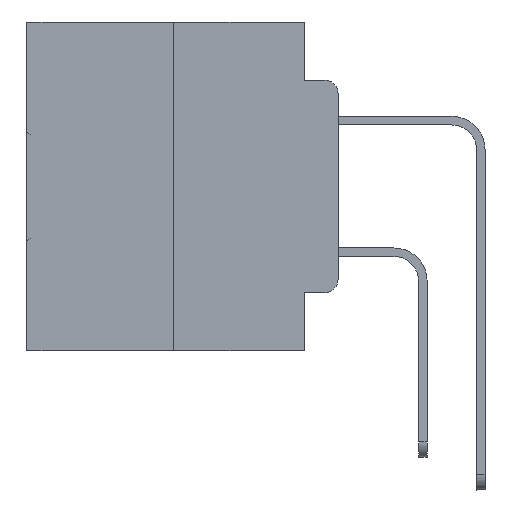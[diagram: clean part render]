
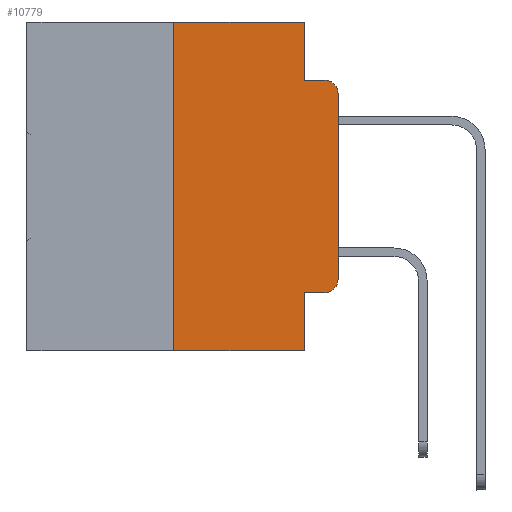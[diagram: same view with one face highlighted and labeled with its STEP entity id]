
A CAD part, left-side view. The second image highlights one B-rep face of the part: STEP entity #10779.
In plain terms, the highlighted planar face has unit normal (-1, 0, 0).
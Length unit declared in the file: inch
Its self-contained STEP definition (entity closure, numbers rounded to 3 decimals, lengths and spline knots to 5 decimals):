
#100 = VERTEX_POINT ( 'NONE', #12382 ) ;
#113 = DIRECTION ( 'NONE',  ( 0., 0., 1. ) ) ;
#302 = LINE ( 'NONE', #7705, #11206 ) ;
#1201 = PLANE ( 'NONE',  #13483 ) ;
#1510 = LINE ( 'NONE', #9770, #7152 ) ;
#1679 = DIRECTION ( 'NONE',  ( 0., -1., 0. ) ) ;
#1878 = CARTESIAN_POINT ( 'NONE',  ( 0., 0.051, 0. ) ) ;
#1931 = VERTEX_POINT ( 'NONE', #5113 ) ;
#3288 = VECTOR ( 'NONE', #32400, 39.37008 ) ;
#3996 = ORIENTED_EDGE ( 'NONE', *, *, #16069, .T. ) ;
#4179 = CARTESIAN_POINT ( 'NONE',  ( 0., 0., -0.1085 ) ) ;
#4691 = VECTOR ( 'NONE', #113, 39.37008 ) ;
#5071 = DIRECTION ( 'NONE',  ( 0., -1., 0. ) ) ;
#5113 = CARTESIAN_POINT ( 'NONE',  ( 0., 0.02, -0.0885 ) ) ;
#5493 = VECTOR ( 'NONE', #5071, 39.37008 ) ;
#6468 = DIRECTION ( 'NONE',  ( 1., 0., 0. ) ) ;
#7084 = CARTESIAN_POINT ( 'NONE',  ( 0., 0.051, -0.4115 ) ) ;
#7152 = VECTOR ( 'NONE', #1679, 39.37008 ) ;
#7705 = CARTESIAN_POINT ( 'NONE',  ( 0., 0., 0. ) ) ;
#8495 = VERTEX_POINT ( 'NONE', #10534 ) ;
#8621 = EDGE_CURVE ( 'NONE', #27660, #28685, #11044, .T. ) ;
#8738 = VERTEX_POINT ( 'NONE', #13031 ) ;
#9267 = DIRECTION ( 'NONE',  ( 0., 0., -1. ) ) ;
#9281 = EDGE_CURVE ( 'NONE', #28875, #8738, #16514, .T. ) ;
#9294 = DIRECTION ( 'NONE',  ( 0., -1., 0. ) ) ;
#9384 = CIRCLE ( 'NONE', #15091, 0.02 ) ;
#9770 = CARTESIAN_POINT ( 'NONE',  ( 0., 0.473, 0. ) ) ;
#9785 = ORIENTED_EDGE ( 'NONE', *, *, #31784, .T. ) ;
#10319 = AXIS2_PLACEMENT_3D ( 'NONE', #24698, #22269, #21919 ) ;
#10534 = CARTESIAN_POINT ( 'NONE',  ( 0., 0.25, -0.5 ) ) ;
#10779 = ADVANCED_FACE ( 'NONE', ( #14029 ), #1201, .F. ) ;
#10921 = VERTEX_POINT ( 'NONE', #4179 ) ;
#11044 = LINE ( 'NONE', #13490, #5493 ) ;
#11206 = VECTOR ( 'NONE', #12969, 39.37008 ) ;
#12021 = ORIENTED_EDGE ( 'NONE', *, *, #8621, .T. ) ;
#12044 = ORIENTED_EDGE ( 'NONE', *, *, #19286, .T. ) ;
#12321 = VECTOR ( 'NONE', #9294, 39.37008 ) ;
#12382 = CARTESIAN_POINT ( 'NONE',  ( 0., 0.051, -0.5 ) ) ;
#12949 = CARTESIAN_POINT ( 'NONE',  ( 0., 0.25, 0. ) ) ;
#12969 = DIRECTION ( 'NONE',  ( 0., 0., 1. ) ) ;
#13020 = ORIENTED_EDGE ( 'NONE', *, *, #25600, .F. ) ;
#13031 = CARTESIAN_POINT ( 'NONE',  ( 0., 0.051, -0.0885 ) ) ;
#13483 = AXIS2_PLACEMENT_3D ( 'NONE', #19846, #6468, #14564 ) ;
#13490 = CARTESIAN_POINT ( 'NONE',  ( 0., 0.051, -0.4115 ) ) ;
#14029 = FACE_OUTER_BOUND ( 'NONE', #25183, .T. ) ;
#14564 = DIRECTION ( 'NONE',  ( 0., 0., -1. ) ) ;
#15088 = DIRECTION ( 'NONE',  ( 0., -1., 0. ) ) ;
#15091 = AXIS2_PLACEMENT_3D ( 'NONE', #34619, #24130, #18386 ) ;
#15795 = CARTESIAN_POINT ( 'NONE',  ( 0., 0.051, -0.0885 ) ) ;
#15839 = CARTESIAN_POINT ( 'NONE',  ( 0., 0., -0.3915 ) ) ;
#16069 = EDGE_CURVE ( 'NONE', #28685, #26930, #21543, .T. ) ;
#16189 = EDGE_CURVE ( 'NONE', #27660, #100, #19995, .T. ) ;
#16393 = LINE ( 'NONE', #29835, #12321 ) ;
#16514 = LINE ( 'NONE', #21760, #3288 ) ;
#18386 = DIRECTION ( 'NONE',  ( 0., 0., -1. ) ) ;
#18611 = CARTESIAN_POINT ( 'NONE',  ( 0., 0.02, -0.4115 ) ) ;
#19183 = ORIENTED_EDGE ( 'NONE', *, *, #9281, .F. ) ;
#19286 = EDGE_CURVE ( 'NONE', #8495, #100, #16393, .T. ) ;
#19310 = VECTOR ( 'NONE', #9267, 39.37008 ) ;
#19402 = VECTOR ( 'NONE', #15088, 39.37008 ) ;
#19473 = ORIENTED_EDGE ( 'NONE', *, *, #30697, .F. ) ;
#19846 = CARTESIAN_POINT ( 'NONE',  ( 0., 0.473, 0. ) ) ;
#19995 = LINE ( 'NONE', #1878, #19310 ) ;
#21051 = LINE ( 'NONE', #15795, #19402 ) ;
#21395 = CARTESIAN_POINT ( 'NONE',  ( 0., 0.051, 0. ) ) ;
#21543 = CIRCLE ( 'NONE', #10319, 0.02 ) ;
#21760 = CARTESIAN_POINT ( 'NONE',  ( 0., 0.051, 0. ) ) ;
#21919 = DIRECTION ( 'NONE',  ( 0., 0., -1. ) ) ;
#22269 = DIRECTION ( 'NONE',  ( -1., 0., 0. ) ) ;
#24130 = DIRECTION ( 'NONE',  ( -1., 0., 0. ) ) ;
#24698 = CARTESIAN_POINT ( 'NONE',  ( 0., 0.02, -0.3915 ) ) ;
#25183 = EDGE_LOOP ( 'NONE', ( #9785, #28261, #31629, #19183, #19473, #13020, #12044, #32175, #12021, #3996 ) ) ;
#25333 = CARTESIAN_POINT ( 'NONE',  ( 0., 0.25, 0. ) ) ;
#25600 = EDGE_CURVE ( 'NONE', #8495, #29361, #26761, .T. ) ;
#26761 = LINE ( 'NONE', #12949, #4691 ) ;
#26930 = VERTEX_POINT ( 'NONE', #15839 ) ;
#27280 = EDGE_CURVE ( 'NONE', #8738, #1931, #21051, .T. ) ;
#27660 = VERTEX_POINT ( 'NONE', #7084 ) ;
#28261 = ORIENTED_EDGE ( 'NONE', *, *, #30882, .T. ) ;
#28685 = VERTEX_POINT ( 'NONE', #18611 ) ;
#28875 = VERTEX_POINT ( 'NONE', #21395 ) ;
#29361 = VERTEX_POINT ( 'NONE', #25333 ) ;
#29835 = CARTESIAN_POINT ( 'NONE',  ( 0., 0.473, -0.5 ) ) ;
#30697 = EDGE_CURVE ( 'NONE', #29361, #28875, #1510, .T. ) ;
#30882 = EDGE_CURVE ( 'NONE', #10921, #1931, #9384, .T. ) ;
#31629 = ORIENTED_EDGE ( 'NONE', *, *, #27280, .F. ) ;
#31784 = EDGE_CURVE ( 'NONE', #26930, #10921, #302, .T. ) ;
#32175 = ORIENTED_EDGE ( 'NONE', *, *, #16189, .F. ) ;
#32400 = DIRECTION ( 'NONE',  ( 0., 0., -1. ) ) ;
#34619 = CARTESIAN_POINT ( 'NONE',  ( 0., 0.02, -0.1085 ) ) ;
